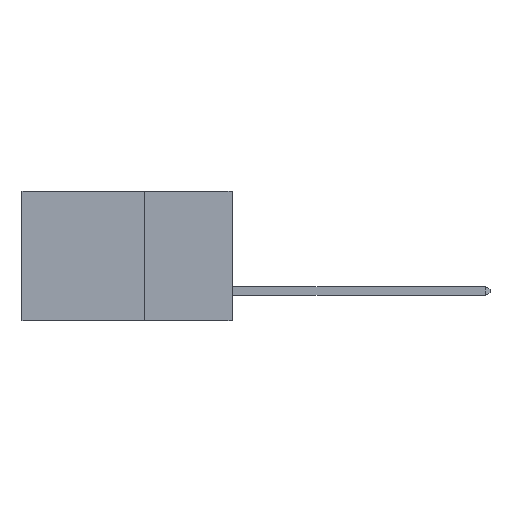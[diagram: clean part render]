
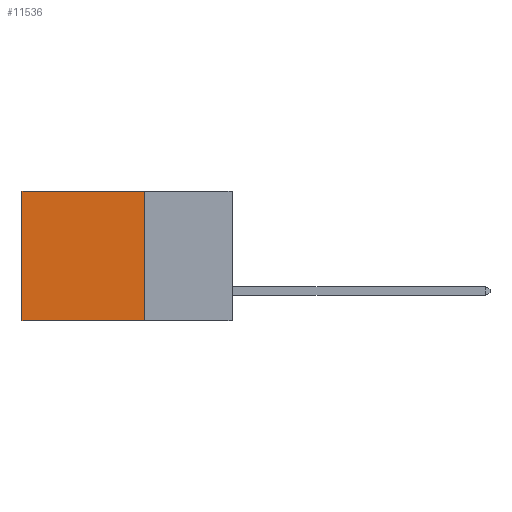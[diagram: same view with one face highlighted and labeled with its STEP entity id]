
A CAD part, left-side view. The second image highlights one B-rep face of the part: STEP entity #11536.
In plain terms, the highlighted planar face has unit normal (-1, 0, 0).
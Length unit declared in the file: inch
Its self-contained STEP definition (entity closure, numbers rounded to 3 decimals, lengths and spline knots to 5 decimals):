
#2818 = ORIENTED_EDGE ( 'NONE', *, *, #25402, .F. ) ;
#3017 = CARTESIAN_POINT ( 'NONE',  ( 0.2875, 0.25, 0. ) ) ;
#3054 = DIRECTION ( 'NONE',  ( 1., 0., 0. ) ) ;
#3311 = DIRECTION ( 'NONE',  ( 0., 0., -1. ) ) ;
#4266 = CARTESIAN_POINT ( 'NONE',  ( 0.2875, 0.6, 0. ) ) ;
#4537 = VECTOR ( 'NONE', #9844, 39.37008 ) ;
#5721 = CARTESIAN_POINT ( 'NONE',  ( 0.2875, 0.6, -0.37 ) ) ;
#5945 = EDGE_CURVE ( 'NONE', #20053, #23084, #9403, .T. ) ;
#5964 = VECTOR ( 'NONE', #24012, 39.37008 ) ;
#7117 = PLANE ( 'NONE',  #25848 ) ;
#8001 = ORIENTED_EDGE ( 'NONE', *, *, #5945, .T. ) ;
#8063 = VERTEX_POINT ( 'NONE', #16991 ) ;
#9403 = LINE ( 'NONE', #22203, #4537 ) ;
#9640 = EDGE_CURVE ( 'NONE', #23084, #15640, #26604, .T. ) ;
#9711 = LINE ( 'NONE', #26235, #26141 ) ;
#9844 = DIRECTION ( 'NONE',  ( 0., 1., 0. ) ) ;
#10199 = VECTOR ( 'NONE', #3311, 39.37008 ) ;
#11536 = ADVANCED_FACE ( 'NONE', ( #19538 ), #7117, .F. ) ;
#11781 = CARTESIAN_POINT ( 'NONE',  ( 0.2875, 0.25, 0. ) ) ;
#11867 = DIRECTION ( 'NONE',  ( 0., 1., 0. ) ) ;
#13402 = CARTESIAN_POINT ( 'NONE',  ( 0.2875, 0.25, 0. ) ) ;
#14002 = ORIENTED_EDGE ( 'NONE', *, *, #22139, .F. ) ;
#15640 = VERTEX_POINT ( 'NONE', #5721 ) ;
#15748 = CARTESIAN_POINT ( 'NONE',  ( 0.2875, 0.6, 0. ) ) ;
#16991 = CARTESIAN_POINT ( 'NONE',  ( 0.2875, 0.25, -0.37 ) ) ;
#17558 = DIRECTION ( 'NONE',  ( 0., 0., -1. ) ) ;
#19538 = FACE_OUTER_BOUND ( 'NONE', #22184, .T. ) ;
#20053 = VERTEX_POINT ( 'NONE', #3017 ) ;
#22139 = EDGE_CURVE ( 'NONE', #8063, #15640, #9711, .T. ) ;
#22184 = EDGE_LOOP ( 'NONE', ( #22238, #14002, #2818, #8001 ) ) ;
#22203 = CARTESIAN_POINT ( 'NONE',  ( 0.2875, 0.25, 0. ) ) ;
#22238 = ORIENTED_EDGE ( 'NONE', *, *, #9640, .T. ) ;
#22422 = LINE ( 'NONE', #11781, #5964 ) ;
#23084 = VERTEX_POINT ( 'NONE', #4266 ) ;
#24012 = DIRECTION ( 'NONE',  ( 0., 0., -1. ) ) ;
#25402 = EDGE_CURVE ( 'NONE', #20053, #8063, #22422, .T. ) ;
#25848 = AXIS2_PLACEMENT_3D ( 'NONE', #13402, #3054, #17558 ) ;
#26141 = VECTOR ( 'NONE', #11867, 39.37008 ) ;
#26235 = CARTESIAN_POINT ( 'NONE',  ( 0.2875, 0.25, -0.37 ) ) ;
#26604 = LINE ( 'NONE', #15748, #10199 ) ;
